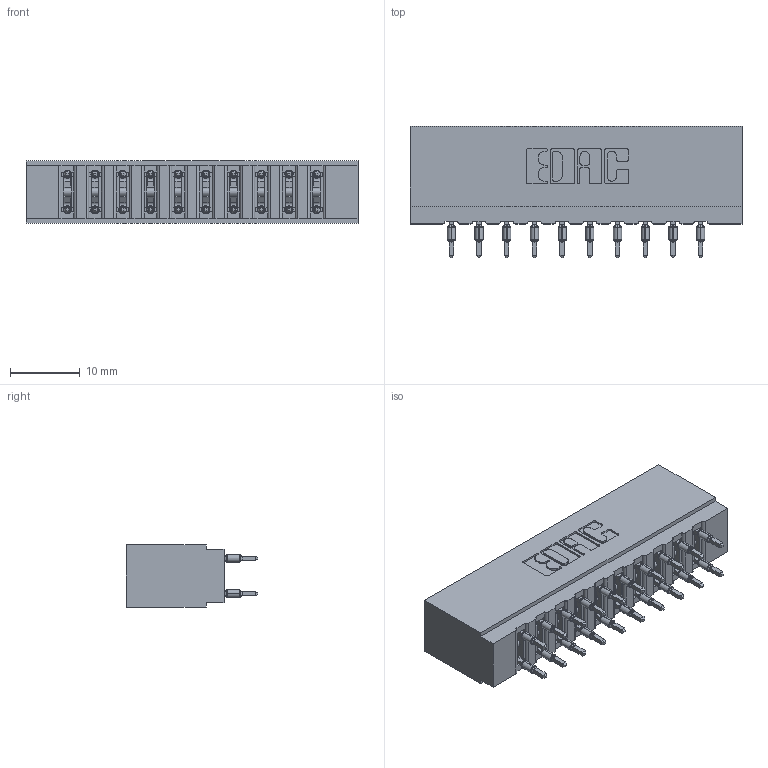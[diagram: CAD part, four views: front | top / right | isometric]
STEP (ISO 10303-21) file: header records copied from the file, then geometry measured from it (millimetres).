
FILE_DESCRIPTION (( 'STEP AP203' ), '1' );
FILE_NAME ('717-020-560-201.STEP', '2026-02-20T17:15:26', ( '' ), ( '' ), 'SwSTEP 2.0', 'SolidWorks 2023', '' );
FILE_SCHEMA (( 'CONFIG_CONTROL_DESIGN' ));
Length unit declared in the file: millimetre
Products named in the file (3): 717 Part_Insulator Option - 06; 717-020-560-201; 745-292-001_560
Assembly tree (21 placements, depth 2):
  717-020-560-201
    717 Part_Insulator Option - 06
    745-292-001_560  x20
Bounding box: 47.5 x 18.78 x 8.89 mm (x, y, z)
Volume: 4321.9 mm3; surface area: 6533.6 mm2
Topology: 21 solids, 21 shells, 2074 faces, 5671 edges, 3606 vertices
Faces by surface type: plane 1084, cylinder 470, bspline 400, torus 120
Entity records: 21788 total; most frequent: CARTESIAN_POINT 4295, ORIENTED_EDGE 3666, DIRECTION 3235, EDGE_CURVE 1833, VECTOR 1583, LINE 1583, VERTEX_POINT 1174, AXIS2_PLACEMENT_3D 826
